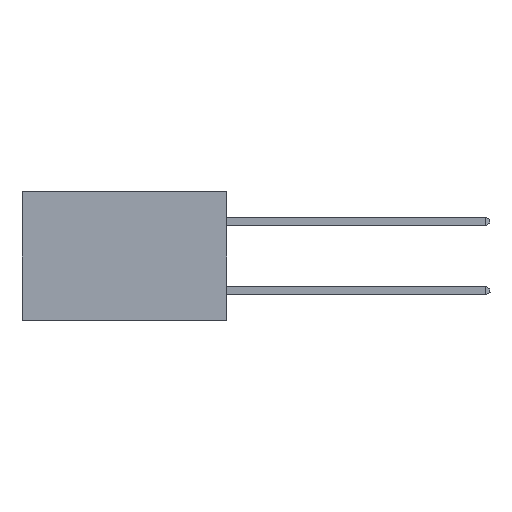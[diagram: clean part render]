
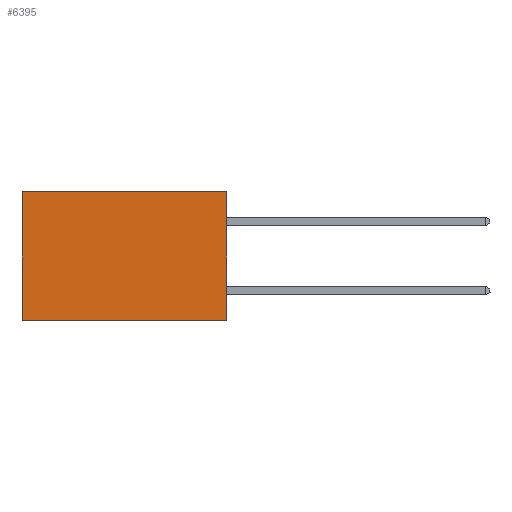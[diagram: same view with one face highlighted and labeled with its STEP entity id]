
A CAD part, left-side view. The second image highlights one B-rep face of the part: STEP entity #6395.
In plain terms, the highlighted planar face has unit normal (-1, 0, 0).
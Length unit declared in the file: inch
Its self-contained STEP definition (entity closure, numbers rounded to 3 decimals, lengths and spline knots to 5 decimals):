
#201 = VERTEX_POINT ( 'NONE', #14853 ) ;
#299 = EDGE_CURVE ( 'NONE', #13510, #4448, #8283, .T. ) ;
#310 = CARTESIAN_POINT ( 'NONE',  ( 0.277, 0., -0.37 ) ) ;
#603 = ORIENTED_EDGE ( 'NONE', *, *, #26074, .F. ) ;
#1288 = DIRECTION ( 'NONE',  ( 0., 1., 0. ) ) ;
#2463 = ORIENTED_EDGE ( 'NONE', *, *, #299, .F. ) ;
#4268 = ORIENTED_EDGE ( 'NONE', *, *, #25123, .T. ) ;
#4448 = VERTEX_POINT ( 'NONE', #6925 ) ;
#6395 = ADVANCED_FACE ( 'NONE', ( #15863 ), #16797, .F. ) ;
#6925 = CARTESIAN_POINT ( 'NONE',  ( 0.277, 0.59, -0.37 ) ) ;
#7094 = VERTEX_POINT ( 'NONE', #14787 ) ;
#7620 = VECTOR ( 'NONE', #26255, 39.37008 ) ;
#8105 = LINE ( 'NONE', #8985, #13786 ) ;
#8283 = LINE ( 'NONE', #26283, #7620 ) ;
#8985 = CARTESIAN_POINT ( 'NONE',  ( 0.277, 0.59, -0.37 ) ) ;
#9722 = EDGE_LOOP ( 'NONE', ( #4268, #2463, #603, #25808 ) ) ;
#11988 = CARTESIAN_POINT ( 'NONE',  ( 0.277, 0., 0. ) ) ;
#13155 = DIRECTION ( 'NONE',  ( 0., 0., -1. ) ) ;
#13510 = VERTEX_POINT ( 'NONE', #26145 ) ;
#13786 = VECTOR ( 'NONE', #19518, 39.37008 ) ;
#14787 = CARTESIAN_POINT ( 'NONE',  ( 0.277, 0.59, 0. ) ) ;
#14853 = CARTESIAN_POINT ( 'NONE',  ( 0.277, 0., 0. ) ) ;
#15863 = FACE_OUTER_BOUND ( 'NONE', #9722, .T. ) ;
#16345 = DIRECTION ( 'NONE',  ( 0., 0., -1. ) ) ;
#16371 = EDGE_CURVE ( 'NONE', #201, #7094, #25858, .T. ) ;
#16432 = CARTESIAN_POINT ( 'NONE',  ( 0.277, 0., -0.37 ) ) ;
#16525 = DIRECTION ( 'NONE',  ( 1., 0., 0. ) ) ;
#16797 = PLANE ( 'NONE',  #19882 ) ;
#18823 = VECTOR ( 'NONE', #13155, 39.37008 ) ;
#19518 = DIRECTION ( 'NONE',  ( 0., 0., -1. ) ) ;
#19882 = AXIS2_PLACEMENT_3D ( 'NONE', #16432, #16525, #16345 ) ;
#20094 = LINE ( 'NONE', #310, #18823 ) ;
#25123 = EDGE_CURVE ( 'NONE', #7094, #4448, #8105, .T. ) ;
#25232 = VECTOR ( 'NONE', #1288, 39.37008 ) ;
#25808 = ORIENTED_EDGE ( 'NONE', *, *, #16371, .T. ) ;
#25858 = LINE ( 'NONE', #11988, #25232 ) ;
#26074 = EDGE_CURVE ( 'NONE', #201, #13510, #20094, .T. ) ;
#26145 = CARTESIAN_POINT ( 'NONE',  ( 0.277, 0., -0.37 ) ) ;
#26255 = DIRECTION ( 'NONE',  ( 0., 1., 0. ) ) ;
#26283 = CARTESIAN_POINT ( 'NONE',  ( 0.277, 0., -0.37 ) ) ;
